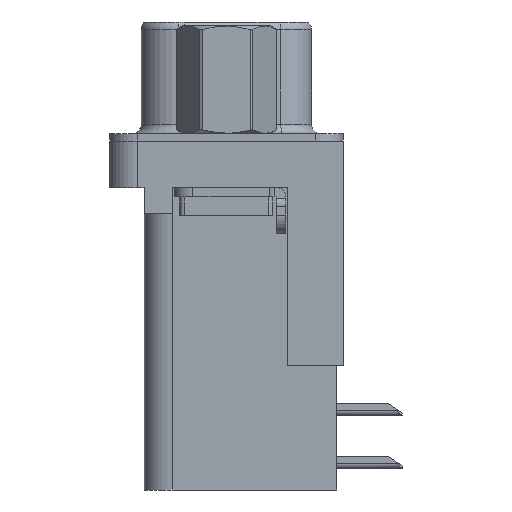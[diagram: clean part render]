
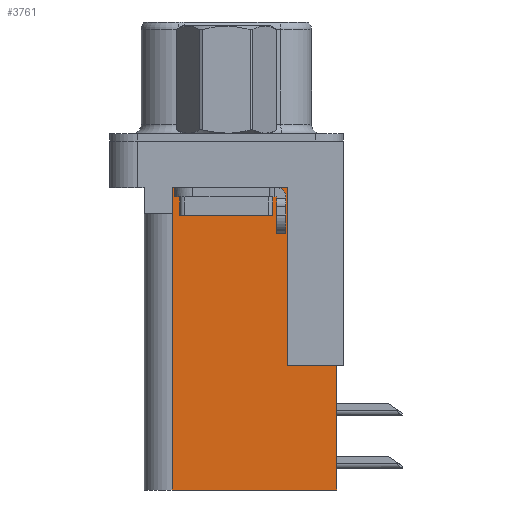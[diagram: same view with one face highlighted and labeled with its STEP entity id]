
A CAD part, left-side view. The second image highlights one B-rep face of the part: STEP entity #3761.
In plain terms, the highlighted planar face has unit normal (-1, 0, 0).
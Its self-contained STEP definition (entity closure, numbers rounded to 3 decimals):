
#149 = CARTESIAN_POINT ( 'NONE',  ( 3.765, 2.925, -3.9 ) ) ;
#453 = EDGE_CURVE ( 'NONE', #11339, #8846, #6115, .T. ) ;
#492 = DIRECTION ( 'NONE',  ( 0., 1., 0. ) ) ;
#1178 = VECTOR ( 'NONE', #15726, 1000. ) ;
#1372 = LINE ( 'NONE', #18033, #1178 ) ;
#2078 = EDGE_CURVE ( 'NONE', #17409, #13734, #1372, .T. ) ;
#2526 = DIRECTION ( 'NONE',  ( 0., 1., 0. ) ) ;
#2579 = DIRECTION ( 'NONE',  ( 1., 0., 0. ) ) ;
#2608 = CARTESIAN_POINT ( 'NONE',  ( 3.765, -3.295, -18.76 ) ) ;
#2765 = EDGE_CURVE ( 'NONE', #14387, #17409, #22968, .T. ) ;
#3100 = PLANE ( 'NONE',  #7795 ) ;
#3118 = CARTESIAN_POINT ( 'NONE',  ( 3.765, 2.925, -18.76 ) ) ;
#3167 = EDGE_CURVE ( 'NONE', #8846, #13734, #21765, .T. ) ;
#3328 = EDGE_LOOP ( 'NONE', ( #11391, #4750, #14252, #21115, #13105, #22251, #3617, #18182 ) ) ;
#3423 = EDGE_CURVE ( 'NONE', #20270, #14387, #20730, .T. ) ;
#3617 = ORIENTED_EDGE ( 'NONE', *, *, #4097, .T. ) ;
#3761 = ADVANCED_FACE ( 'NONE', ( #19306 ), #3100, .F. ) ;
#4097 = EDGE_CURVE ( 'NONE', #20270, #14859, #18060, .T. ) ;
#4550 = EDGE_CURVE ( 'NONE', #14859, #5615, #15662, .T. ) ;
#4750 = ORIENTED_EDGE ( 'NONE', *, *, #453, .T. ) ;
#5114 = VECTOR ( 'NONE', #492, 1000. ) ;
#5191 = LINE ( 'NONE', #13801, #5114 ) ;
#5615 = VERTEX_POINT ( 'NONE', #5804 ) ;
#5804 = CARTESIAN_POINT ( 'NONE',  ( 3.765, -3.295, -2.5 ) ) ;
#5974 = VECTOR ( 'NONE', #22230, 1000. ) ;
#6115 = LINE ( 'NONE', #22306, #5974 ) ;
#7795 = AXIS2_PLACEMENT_3D ( 'NONE', #2608, #2579, #2526 ) ;
#8846 = VERTEX_POINT ( 'NONE', #15133 ) ;
#10658 = CARTESIAN_POINT ( 'NONE',  ( 3.765, -3.295, -18.76 ) ) ;
#11339 = VERTEX_POINT ( 'NONE', #13058 ) ;
#11391 = ORIENTED_EDGE ( 'NONE', *, *, #21214, .T. ) ;
#13058 = CARTESIAN_POINT ( 'NONE',  ( 3.765, 2.895, -2.5 ) ) ;
#13105 = ORIENTED_EDGE ( 'NONE', *, *, #2765, .F. ) ;
#13734 = VERTEX_POINT ( 'NONE', #149 ) ;
#13801 = CARTESIAN_POINT ( 'NONE',  ( 3.765, -3.295, -2.5 ) ) ;
#14252 = ORIENTED_EDGE ( 'NONE', *, *, #3167, .T. ) ;
#14387 = VERTEX_POINT ( 'NONE', #21994 ) ;
#14449 = DIRECTION ( 'NONE',  ( 0., 0., 1. ) ) ;
#14859 = VERTEX_POINT ( 'NONE', #21437 ) ;
#15133 = CARTESIAN_POINT ( 'NONE',  ( 3.765, 2.895, -3.9 ) ) ;
#15141 = CARTESIAN_POINT ( 'NONE',  ( 3.765, -3.295, -18.76 ) ) ;
#15599 = VECTOR ( 'NONE', #14449, 1000. ) ;
#15662 = LINE ( 'NONE', #15141, #15599 ) ;
#15726 = DIRECTION ( 'NONE',  ( 0., 0., 1. ) ) ;
#17409 = VERTEX_POINT ( 'NONE', #3118 ) ;
#17875 = VECTOR ( 'NONE', #22997, 1000. ) ;
#18033 = CARTESIAN_POINT ( 'NONE',  ( 3.765, 2.925, -18.76 ) ) ;
#18060 = LINE ( 'NONE', #23108, #17875 ) ;
#18182 = ORIENTED_EDGE ( 'NONE', *, *, #4550, .T. ) ;
#19306 = FACE_OUTER_BOUND ( 'NONE', #3328, .T. ) ;
#20264 = CARTESIAN_POINT ( 'NONE',  ( 3.765, -5.925, -12.05 ) ) ;
#20270 = VERTEX_POINT ( 'NONE', #20264 ) ;
#20328 = DIRECTION ( 'NONE',  ( 0., 1., 0. ) ) ;
#20708 = VECTOR ( 'NONE', #23298, 1000. ) ;
#20730 = LINE ( 'NONE', #23493, #20708 ) ;
#21115 = ORIENTED_EDGE ( 'NONE', *, *, #2078, .F. ) ;
#21214 = EDGE_CURVE ( 'NONE', #5615, #11339, #5191, .T. ) ;
#21437 = CARTESIAN_POINT ( 'NONE',  ( 3.765, -3.295, -12.05 ) ) ;
#21615 = CARTESIAN_POINT ( 'NONE',  ( 3.765, 0., -3.9 ) ) ;
#21765 = LINE ( 'NONE', #21615, #21807 ) ;
#21807 = VECTOR ( 'NONE', #20328, 1000. ) ;
#21881 = DIRECTION ( 'NONE',  ( 0., 1., 0. ) ) ;
#21994 = CARTESIAN_POINT ( 'NONE',  ( 3.765, -5.925, -18.76 ) ) ;
#22230 = DIRECTION ( 'NONE',  ( 0., 0., -1. ) ) ;
#22251 = ORIENTED_EDGE ( 'NONE', *, *, #3423, .F. ) ;
#22306 = CARTESIAN_POINT ( 'NONE',  ( 3.765, 2.895, -3.9 ) ) ;
#22946 = VECTOR ( 'NONE', #21881, 1000. ) ;
#22968 = LINE ( 'NONE', #10658, #22946 ) ;
#22997 = DIRECTION ( 'NONE',  ( 0., 1., 0. ) ) ;
#23108 = CARTESIAN_POINT ( 'NONE',  ( 3.765, -6.295, -12.05 ) ) ;
#23298 = DIRECTION ( 'NONE',  ( 0., 0., -1. ) ) ;
#23493 = CARTESIAN_POINT ( 'NONE',  ( 3.765, -5.925, -2. ) ) ;
